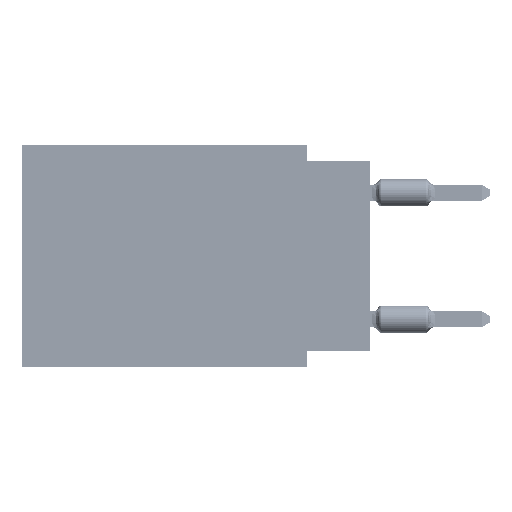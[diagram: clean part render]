
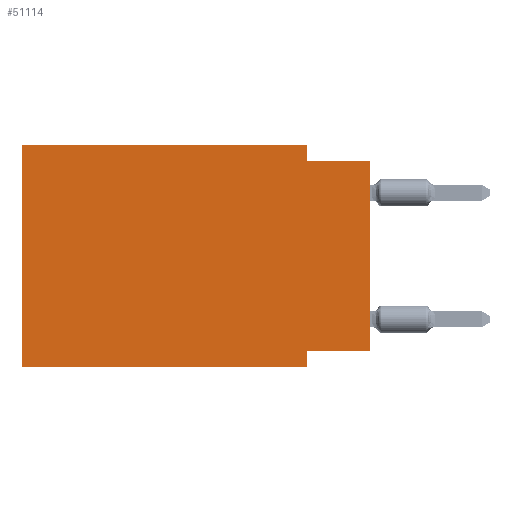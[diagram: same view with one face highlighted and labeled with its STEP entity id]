
A CAD part, left-side view. The second image highlights one B-rep face of the part: STEP entity #51114.
In plain terms, the highlighted planar face has unit normal (-1, 0, 0).
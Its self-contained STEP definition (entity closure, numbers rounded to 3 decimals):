
#56 = DIRECTION ( 'NONE',  ( 0., 0., -1. ) ) ;
#209 = VECTOR ( 'NONE', #56, 1000. ) ;
#1550 = CARTESIAN_POINT ( 'NONE',  ( 0., 13.97, -8.89 ) ) ;
#2621 = CARTESIAN_POINT ( 'NONE',  ( 0., 2.54, -8.89 ) ) ;
#4136 = DIRECTION ( 'NONE',  ( 0., -1., 0. ) ) ;
#4161 = CARTESIAN_POINT ( 'NONE',  ( 0., 0., -0.635 ) ) ;
#5075 = EDGE_CURVE ( 'NONE', #14818, #44073, #49707, .T. ) ;
#7920 = EDGE_CURVE ( 'NONE', #21042, #14818, #29587, .T. ) ;
#8960 = DIRECTION ( 'NONE',  ( 1., 0., 0. ) ) ;
#10654 = ORIENTED_EDGE ( 'NONE', *, *, #5075, .F. ) ;
#10716 = LINE ( 'NONE', #28811, #54625 ) ;
#11640 = VECTOR ( 'NONE', #19878, 1000. ) ;
#12275 = VERTEX_POINT ( 'NONE', #22802 ) ;
#14305 = CARTESIAN_POINT ( 'NONE',  ( 0., 2.54, -8.89 ) ) ;
#14323 = CARTESIAN_POINT ( 'NONE',  ( 0., 0., -8.255 ) ) ;
#14818 = VERTEX_POINT ( 'NONE', #31517 ) ;
#15420 = LINE ( 'NONE', #42425, #11640 ) ;
#18954 = CARTESIAN_POINT ( 'NONE',  ( 0., 2.54, 0. ) ) ;
#19878 = DIRECTION ( 'NONE',  ( 0., 0., 1. ) ) ;
#20418 = DIRECTION ( 'NONE',  ( 0., 0., 1. ) ) ;
#20724 = EDGE_CURVE ( 'NONE', #21042, #50089, #52293, .T. ) ;
#21042 = VERTEX_POINT ( 'NONE', #1550 ) ;
#22802 = CARTESIAN_POINT ( 'NONE',  ( 0., 0., -8.255 ) ) ;
#24258 = CARTESIAN_POINT ( 'NONE',  ( 0., 13.97, 0. ) ) ;
#24824 = ORIENTED_EDGE ( 'NONE', *, *, #20724, .T. ) ;
#24940 = CARTESIAN_POINT ( 'NONE',  ( 0., 2.54, -8.255 ) ) ;
#26979 = EDGE_CURVE ( 'NONE', #36129, #50089, #41302, .T. ) ;
#27397 = DIRECTION ( 'NONE',  ( 0., 1., 0. ) ) ;
#28024 = ORIENTED_EDGE ( 'NONE', *, *, #44999, .F. ) ;
#28811 = CARTESIAN_POINT ( 'NONE',  ( 0., 0., -0.635 ) ) ;
#29587 = LINE ( 'NONE', #24258, #50580 ) ;
#31517 = CARTESIAN_POINT ( 'NONE',  ( 0., 13.97, 0. ) ) ;
#32238 = VECTOR ( 'NONE', #57637, 1000. ) ;
#32998 = DIRECTION ( 'NONE',  ( 0., 0., -1. ) ) ;
#33781 = ORIENTED_EDGE ( 'NONE', *, *, #7920, .F. ) ;
#34094 = EDGE_CURVE ( 'NONE', #12275, #36129, #50790, .T. ) ;
#35083 = DIRECTION ( 'NONE',  ( 0., 0., -1. ) ) ;
#35952 = FACE_OUTER_BOUND ( 'NONE', #54237, .T. ) ;
#36129 = VERTEX_POINT ( 'NONE', #24940 ) ;
#37292 = EDGE_CURVE ( 'NONE', #48656, #46500, #10716, .T. ) ;
#38210 = VECTOR ( 'NONE', #58319, 1000. ) ;
#39280 = CARTESIAN_POINT ( 'NONE',  ( 0., 13.97, -8.89 ) ) ;
#41302 = LINE ( 'NONE', #14305, #42478 ) ;
#41887 = VECTOR ( 'NONE', #27397, 1000. ) ;
#42425 = CARTESIAN_POINT ( 'NONE',  ( 0., 0., 0. ) ) ;
#42478 = VECTOR ( 'NONE', #32998, 1000. ) ;
#44073 = VERTEX_POINT ( 'NONE', #18954 ) ;
#44507 = ORIENTED_EDGE ( 'NONE', *, *, #37292, .F. ) ;
#44999 = EDGE_CURVE ( 'NONE', #44073, #48656, #49578, .T. ) ;
#45135 = PLANE ( 'NONE',  #57345 ) ;
#45441 = ORIENTED_EDGE ( 'NONE', *, *, #48000, .T. ) ;
#46500 = VERTEX_POINT ( 'NONE', #4161 ) ;
#48000 = EDGE_CURVE ( 'NONE', #12275, #46500, #15420, .T. ) ;
#48656 = VERTEX_POINT ( 'NONE', #49193 ) ;
#49131 = CARTESIAN_POINT ( 'NONE',  ( 0., 13.97, 0. ) ) ;
#49193 = CARTESIAN_POINT ( 'NONE',  ( 0., 2.54, -0.635 ) ) ;
#49578 = LINE ( 'NONE', #55178, #209 ) ;
#49707 = LINE ( 'NONE', #49131, #38210 ) ;
#50089 = VERTEX_POINT ( 'NONE', #2621 ) ;
#50580 = VECTOR ( 'NONE', #20418, 1000. ) ;
#50790 = LINE ( 'NONE', #14323, #41887 ) ;
#51114 = ADVANCED_FACE ( 'NONE', ( #35952 ), #45135, .F. ) ;
#52293 = LINE ( 'NONE', #39280, #32238 ) ;
#52857 = CARTESIAN_POINT ( 'NONE',  ( 0., 13.97, 0. ) ) ;
#53606 = ORIENTED_EDGE ( 'NONE', *, *, #26979, .F. ) ;
#54237 = EDGE_LOOP ( 'NONE', ( #45441, #44507, #28024, #10654, #33781, #24824, #53606, #54446 ) ) ;
#54446 = ORIENTED_EDGE ( 'NONE', *, *, #34094, .F. ) ;
#54625 = VECTOR ( 'NONE', #4136, 1000. ) ;
#55178 = CARTESIAN_POINT ( 'NONE',  ( 0., 2.54, 0. ) ) ;
#57345 = AXIS2_PLACEMENT_3D ( 'NONE', #52857, #8960, #35083 ) ;
#57637 = DIRECTION ( 'NONE',  ( 0., -1., 0. ) ) ;
#58319 = DIRECTION ( 'NONE',  ( 0., -1., 0. ) ) ;
